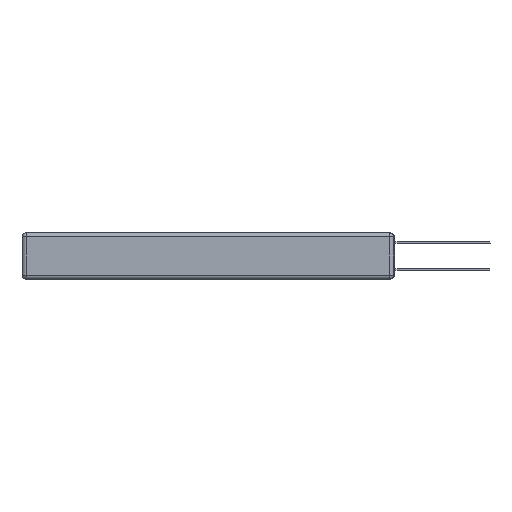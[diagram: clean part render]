
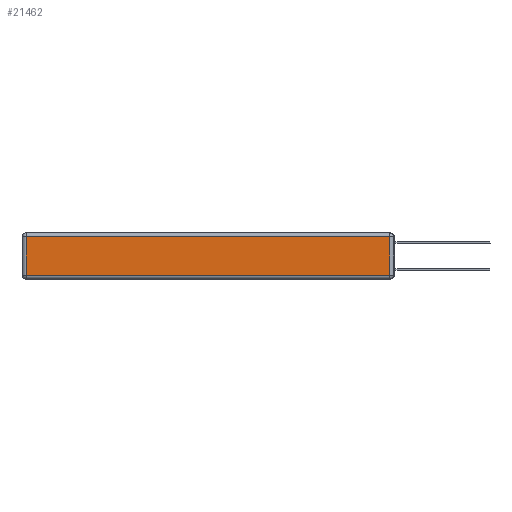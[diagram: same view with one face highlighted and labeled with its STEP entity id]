
A CAD part, left-side view. The second image highlights one B-rep face of the part: STEP entity #21462.
In plain terms, the highlighted planar face has unit normal (-1, 0, 0).
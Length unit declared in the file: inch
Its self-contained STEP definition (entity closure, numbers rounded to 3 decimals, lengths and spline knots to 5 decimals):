
#1216 = VERTEX_POINT ( 'NONE', #11048 ) ;
#2341 = VERTEX_POINT ( 'NONE', #17292 ) ;
#3468 = LINE ( 'NONE', #3615, #20163 ) ;
#3602 = CARTESIAN_POINT ( 'NONE',  ( 0., 0., -0.313 ) ) ;
#3615 = CARTESIAN_POINT ( 'NONE',  ( 0., 0.03, -0.343 ) ) ;
#4030 = DIRECTION ( 'NONE',  ( 0., 0., -1. ) ) ;
#4812 = ORIENTED_EDGE ( 'NONE', *, *, #7899, .T. ) ;
#4956 = AXIS2_PLACEMENT_3D ( 'NONE', #20519, #25063, #20926 ) ;
#6195 = VECTOR ( 'NONE', #20522, 39.37008 ) ;
#7852 = DIRECTION ( 'NONE',  ( 0., -1., 0. ) ) ;
#7899 = EDGE_CURVE ( 'NONE', #13061, #1216, #19080, .T. ) ;
#8184 = VECTOR ( 'NONE', #4030, 39.37008 ) ;
#9588 = CARTESIAN_POINT ( 'NONE',  ( 0., 2.75, -0.03 ) ) ;
#9811 = EDGE_LOOP ( 'NONE', ( #13657, #23985, #19958, #4812 ) ) ;
#9951 = EDGE_CURVE ( 'NONE', #2341, #13061, #26582, .T. ) ;
#10562 = CARTESIAN_POINT ( 'NONE',  ( 0., 2.72, -0.03 ) ) ;
#11048 = CARTESIAN_POINT ( 'NONE',  ( 0., 2.72, -0.313 ) ) ;
#12657 = CARTESIAN_POINT ( 'NONE',  ( 0., 2.72, -0.343 ) ) ;
#13061 = VERTEX_POINT ( 'NONE', #10562 ) ;
#13657 = ORIENTED_EDGE ( 'NONE', *, *, #22656, .T. ) ;
#13835 = VERTEX_POINT ( 'NONE', #26529 ) ;
#14253 = PLANE ( 'NONE',  #4956 ) ;
#14366 = EDGE_CURVE ( 'NONE', #13835, #2341, #3468, .T. ) ;
#15521 = VECTOR ( 'NONE', #7852, 39.37008 ) ;
#16972 = FACE_OUTER_BOUND ( 'NONE', #9811, .T. ) ;
#17292 = CARTESIAN_POINT ( 'NONE',  ( 0., 0.03, -0.03 ) ) ;
#18551 = DIRECTION ( 'NONE',  ( 0., 0., 1. ) ) ;
#19080 = LINE ( 'NONE', #12657, #8184 ) ;
#19958 = ORIENTED_EDGE ( 'NONE', *, *, #9951, .T. ) ;
#20163 = VECTOR ( 'NONE', #18551, 39.37008 ) ;
#20519 = CARTESIAN_POINT ( 'NONE',  ( 0., 0., -0.343 ) ) ;
#20522 = DIRECTION ( 'NONE',  ( 0., 1., 0. ) ) ;
#20926 = DIRECTION ( 'NONE',  ( 0., 0., 1. ) ) ;
#21462 = ADVANCED_FACE ( 'NONE', ( #16972 ), #14253, .T. ) ;
#22656 = EDGE_CURVE ( 'NONE', #1216, #13835, #22764, .T. ) ;
#22764 = LINE ( 'NONE', #3602, #15521 ) ;
#23985 = ORIENTED_EDGE ( 'NONE', *, *, #14366, .T. ) ;
#25063 = DIRECTION ( 'NONE',  ( -1., 0., 0. ) ) ;
#26529 = CARTESIAN_POINT ( 'NONE',  ( 0., 0.03, -0.313 ) ) ;
#26582 = LINE ( 'NONE', #9588, #6195 ) ;
